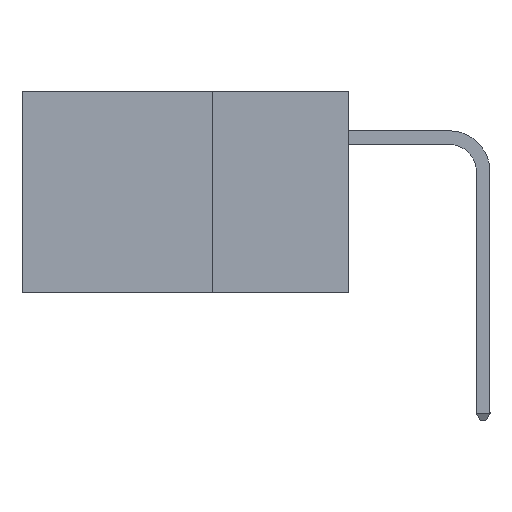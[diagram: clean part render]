
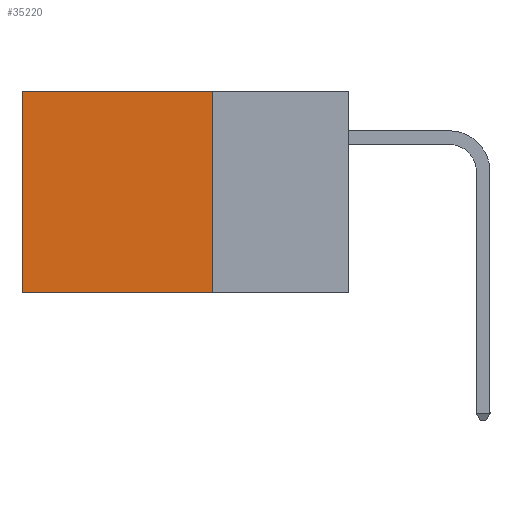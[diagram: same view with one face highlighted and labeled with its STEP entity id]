
A CAD part, left-side view. The second image highlights one B-rep face of the part: STEP entity #35220.
In plain terms, the highlighted planar face has unit normal (-1, 0, 0).
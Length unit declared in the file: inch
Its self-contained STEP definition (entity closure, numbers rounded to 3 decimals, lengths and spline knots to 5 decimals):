
#920 = CARTESIAN_POINT ( 'NONE',  ( 0.2875, 0.6, 0. ) ) ;
#3658 = LINE ( 'NONE', #32162, #32863 ) ;
#4764 = EDGE_LOOP ( 'NONE', ( #30245, #11837, #25115, #8510 ) ) ;
#5967 = LINE ( 'NONE', #19464, #27888 ) ;
#7078 = LINE ( 'NONE', #27725, #12461 ) ;
#7827 = DIRECTION ( 'NONE',  ( 0., 0., -1. ) ) ;
#8035 = DIRECTION ( 'NONE',  ( 0., 0., -1. ) ) ;
#8510 = ORIENTED_EDGE ( 'NONE', *, *, #16920, .T. ) ;
#8812 = EDGE_CURVE ( 'NONE', #20906, #23387, #7078, .T. ) ;
#10478 = DIRECTION ( 'NONE',  ( 1., 0., 0. ) ) ;
#10662 = LINE ( 'NONE', #33557, #17115 ) ;
#11410 = DIRECTION ( 'NONE',  ( 0., 1., 0. ) ) ;
#11837 = ORIENTED_EDGE ( 'NONE', *, *, #25468, .F. ) ;
#12461 = VECTOR ( 'NONE', #7827, 39.37008 ) ;
#13738 = VERTEX_POINT ( 'NONE', #34507 ) ;
#15223 = EDGE_CURVE ( 'NONE', #21371, #13738, #10662, .T. ) ;
#16920 = EDGE_CURVE ( 'NONE', #21371, #20906, #5967, .T. ) ;
#17115 = VECTOR ( 'NONE', #27006, 39.37008 ) ;
#19464 = CARTESIAN_POINT ( 'NONE',  ( 0.2875, 0.25, 0. ) ) ;
#20114 = AXIS2_PLACEMENT_3D ( 'NONE', #30579, #10478, #8035 ) ;
#20906 = VERTEX_POINT ( 'NONE', #920 ) ;
#21371 = VERTEX_POINT ( 'NONE', #30321 ) ;
#23387 = VERTEX_POINT ( 'NONE', #32512 ) ;
#24363 = PLANE ( 'NONE',  #20114 ) ;
#25115 = ORIENTED_EDGE ( 'NONE', *, *, #15223, .F. ) ;
#25468 = EDGE_CURVE ( 'NONE', #13738, #23387, #3658, .T. ) ;
#27006 = DIRECTION ( 'NONE',  ( 0., 0., -1. ) ) ;
#27725 = CARTESIAN_POINT ( 'NONE',  ( 0.2875, 0.6, 0. ) ) ;
#27888 = VECTOR ( 'NONE', #11410, 39.37008 ) ;
#29362 = DIRECTION ( 'NONE',  ( 0., 1., 0. ) ) ;
#30189 = FACE_OUTER_BOUND ( 'NONE', #4764, .T. ) ;
#30245 = ORIENTED_EDGE ( 'NONE', *, *, #8812, .T. ) ;
#30321 = CARTESIAN_POINT ( 'NONE',  ( 0.2875, 0.25, 0. ) ) ;
#30579 = CARTESIAN_POINT ( 'NONE',  ( 0.2875, 0.25, 0. ) ) ;
#32162 = CARTESIAN_POINT ( 'NONE',  ( 0.2875, 0.25, -0.37 ) ) ;
#32512 = CARTESIAN_POINT ( 'NONE',  ( 0.2875, 0.6, -0.37 ) ) ;
#32863 = VECTOR ( 'NONE', #29362, 39.37008 ) ;
#33557 = CARTESIAN_POINT ( 'NONE',  ( 0.2875, 0.25, 0. ) ) ;
#34507 = CARTESIAN_POINT ( 'NONE',  ( 0.2875, 0.25, -0.37 ) ) ;
#35220 = ADVANCED_FACE ( 'NONE', ( #30189 ), #24363, .F. ) ;
